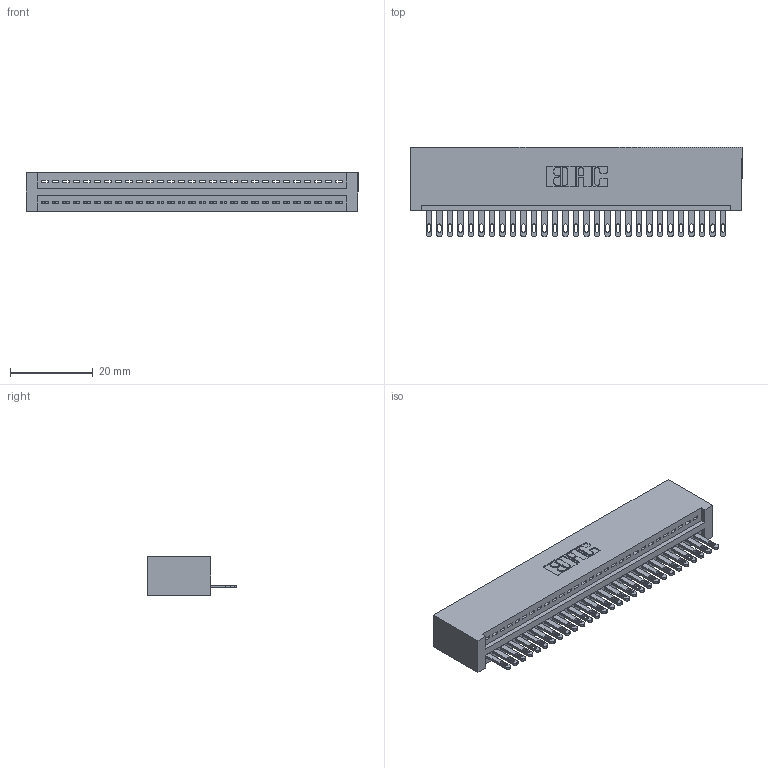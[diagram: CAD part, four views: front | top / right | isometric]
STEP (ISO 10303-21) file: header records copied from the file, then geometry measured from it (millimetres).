
FILE_DESCRIPTION (( 'STEP AP203' ), '1' );
FILE_NAME ('345-029-500-101.STEP', '2019-10-07T06:36:41', ( '' ), ( '' ), 'SwSTEP 2.0', 'SolidWorks 2016', '' );
FILE_SCHEMA (( 'CONFIG_CONTROL_DESIGN' ));
Length unit declared in the file: inch
Products named in the file (3): 345-029-500-101; 345 Part_No Mounting Lugs; 345-292-001_345-293-100
Assembly tree (30 placements, depth 2):
  345-029-500-101
    345 Part_No Mounting Lugs
    345-292-001_345-293-100  x29
Bounding box: 80.26 x 21.51 x 9.4 mm (x, y, z)
Volume: 8119.4 mm3; surface area: 10868.5 mm2
Topology: 30 solids, 30 shells, 1684 faces, 5189 edges, 3458 vertices
Faces by surface type: plane 1062, cylinder 622
Entity records: 23229 total; most frequent: CARTESIAN_POINT 4031, ORIENTED_EDGE 3994, DIRECTION 3535, EDGE_CURVE 1997, VECTOR 1753, LINE 1753, VERTEX_POINT 1330, AXIS2_PLACEMENT_3D 891
